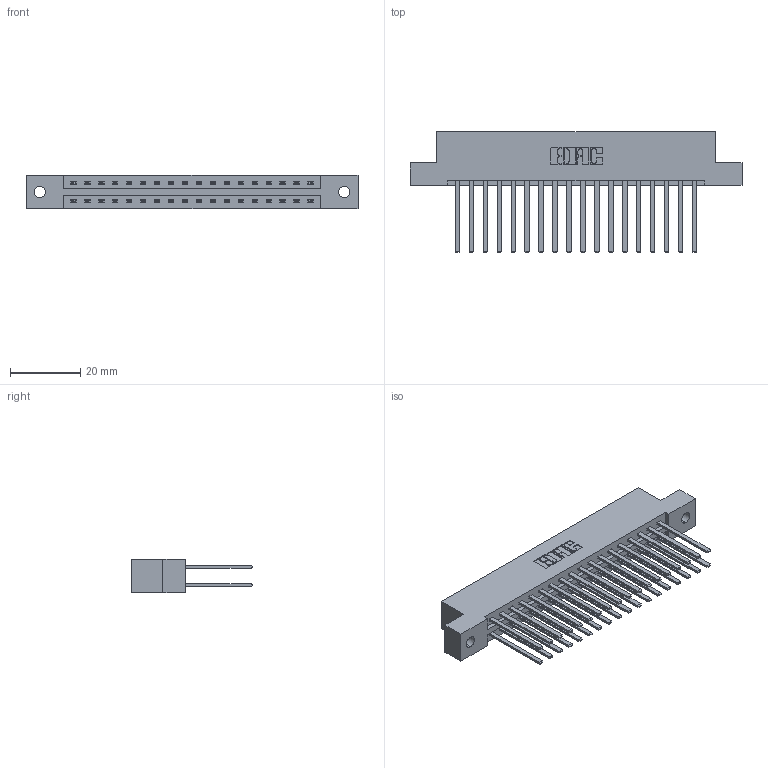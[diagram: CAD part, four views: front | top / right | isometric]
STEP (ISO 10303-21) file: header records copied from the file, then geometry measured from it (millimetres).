
FILE_DESCRIPTION (( 'STEP AP203' ), '1' );
FILE_NAME ('337-036-544-202.STEP', '2018-08-07T23:29:37', ( '' ), ( '' ), 'SwSTEP 2.0', 'SolidWorks 2016', '' );
FILE_SCHEMA (( 'CONFIG_CONTROL_DESIGN' ));
Length unit declared in the file: inch
Products named in the file (3): 337 Part_Flush Mounting Lugs - 0.128 Dia; 345-292-001_345-293-144; 337-036-544-202
Assembly tree (37 placements, depth 2):
  337-036-544-202
    337 Part_Flush Mounting Lugs - 0.128 Dia
    345-292-001_345-293-144  x36
Bounding box: 94.34 x 34.3 x 9.4 mm (x, y, z)
Volume: 10090.3 mm3; surface area: 12549.9 mm2
Topology: 37 solids, 37 shells, 1842 faces, 5459 edges, 3590 vertices
Faces by surface type: plane 1294, cylinder 548
Entity records: 16879 total; most frequent: CARTESIAN_POINT 2862, ORIENTED_EDGE 2798, DIRECTION 2475, EDGE_CURVE 1399, VECTOR 1275, LINE 1275, VERTEX_POINT 930, AXIS2_PLACEMENT_3D 600
